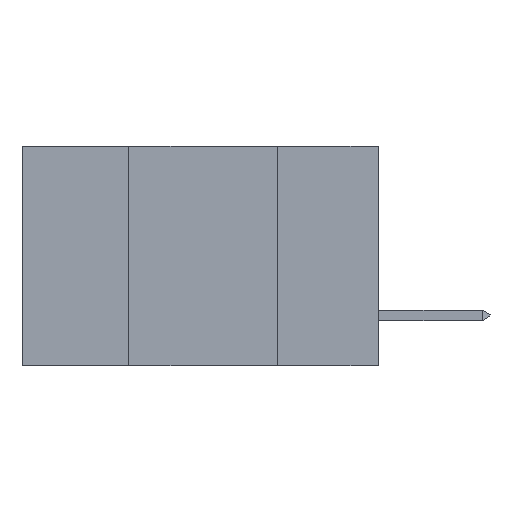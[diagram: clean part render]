
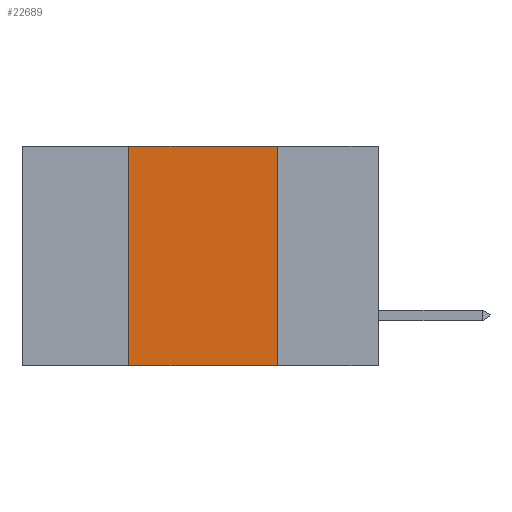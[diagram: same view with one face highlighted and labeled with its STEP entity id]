
A CAD part, left-side view. The second image highlights one B-rep face of the part: STEP entity #22689.
In plain terms, the highlighted planar face has unit normal (-1, 0, 0).
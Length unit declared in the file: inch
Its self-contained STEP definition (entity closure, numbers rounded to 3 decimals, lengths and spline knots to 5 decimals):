
#729 = VECTOR ( 'NONE', #26976, 39.37008 ) ;
#787 = AXIS2_PLACEMENT_3D ( 'NONE', #19021, #18917, #13913 ) ;
#1432 = VERTEX_POINT ( 'NONE', #30050 ) ;
#1841 = EDGE_LOOP ( 'NONE', ( #19137, #21954, #5259, #6356 ) ) ;
#3520 = LINE ( 'NONE', #8344, #27046 ) ;
#5259 = ORIENTED_EDGE ( 'NONE', *, *, #5579, .F. ) ;
#5534 = LINE ( 'NONE', #9895, #29102 ) ;
#5579 = EDGE_CURVE ( 'NONE', #15404, #12926, #3520, .T. ) ;
#6356 = ORIENTED_EDGE ( 'NONE', *, *, #11163, .T. ) ;
#8344 = CARTESIAN_POINT ( 'NONE',  ( 0., 0.42, 0. ) ) ;
#9895 = CARTESIAN_POINT ( 'NONE',  ( 0., 0.6, 0. ) ) ;
#11163 = EDGE_CURVE ( 'NONE', #15404, #30814, #21365, .T. ) ;
#11679 = CARTESIAN_POINT ( 'NONE',  ( 0., 0.17, -0.37 ) ) ;
#12926 = VERTEX_POINT ( 'NONE', #19808 ) ;
#13227 = DIRECTION ( 'NONE',  ( 0., 0., 1. ) ) ;
#13913 = DIRECTION ( 'NONE',  ( 0., 0., -1. ) ) ;
#13982 = EDGE_CURVE ( 'NONE', #12926, #1432, #5534, .T. ) ;
#14850 = VECTOR ( 'NONE', #29539, 39.37008 ) ;
#15404 = VERTEX_POINT ( 'NONE', #26157 ) ;
#17120 = CARTESIAN_POINT ( 'NONE',  ( 0., 0.17, 0. ) ) ;
#18917 = DIRECTION ( 'NONE',  ( 1., 0., 0. ) ) ;
#19021 = CARTESIAN_POINT ( 'NONE',  ( 0., 0.6, 0. ) ) ;
#19123 = PLANE ( 'NONE',  #787 ) ;
#19137 = ORIENTED_EDGE ( 'NONE', *, *, #19800, .F. ) ;
#19800 = EDGE_CURVE ( 'NONE', #1432, #30814, #28055, .T. ) ;
#19808 = CARTESIAN_POINT ( 'NONE',  ( 0., 0.42, 0. ) ) ;
#21365 = LINE ( 'NONE', #24677, #14850 ) ;
#21954 = ORIENTED_EDGE ( 'NONE', *, *, #13982, .F. ) ;
#22689 = ADVANCED_FACE ( 'NONE', ( #25870 ), #19123, .F. ) ;
#24677 = CARTESIAN_POINT ( 'NONE',  ( 0., 0.6, -0.37 ) ) ;
#25870 = FACE_OUTER_BOUND ( 'NONE', #1841, .T. ) ;
#26157 = CARTESIAN_POINT ( 'NONE',  ( 0., 0.42, -0.37 ) ) ;
#26566 = DIRECTION ( 'NONE',  ( 0., -1., 0. ) ) ;
#26976 = DIRECTION ( 'NONE',  ( 0., 0., -1. ) ) ;
#27046 = VECTOR ( 'NONE', #13227, 39.37008 ) ;
#28055 = LINE ( 'NONE', #17120, #729 ) ;
#29102 = VECTOR ( 'NONE', #26566, 39.37008 ) ;
#29539 = DIRECTION ( 'NONE',  ( 0., -1., 0. ) ) ;
#30050 = CARTESIAN_POINT ( 'NONE',  ( 0., 0.17, 0. ) ) ;
#30814 = VERTEX_POINT ( 'NONE', #11679 ) ;
